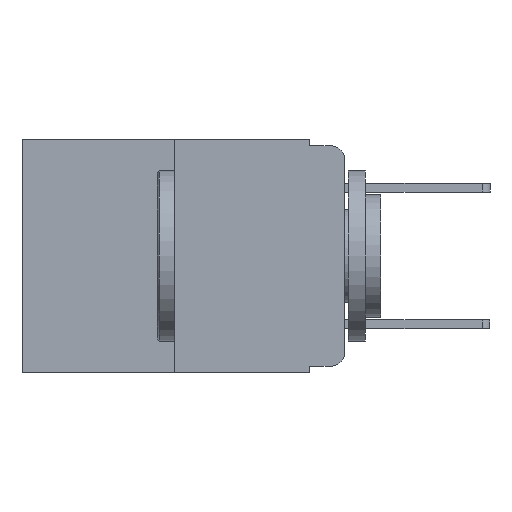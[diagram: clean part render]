
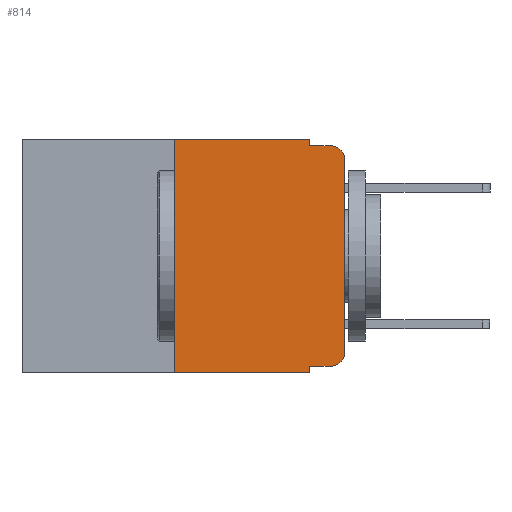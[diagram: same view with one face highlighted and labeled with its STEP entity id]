
A CAD part, left-side view. The second image highlights one B-rep face of the part: STEP entity #814.
In plain terms, the highlighted planar face has unit normal (-1, 0, 0).
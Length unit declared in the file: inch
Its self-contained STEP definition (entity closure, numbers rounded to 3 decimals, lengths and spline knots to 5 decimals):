
#743 = LINE ( 'NONE', #25751, #10506 ) ;
#814 = ADVANCED_FACE ( 'NONE', ( #19289 ), #8830, .F. ) ;
#1158 = CARTESIAN_POINT ( 'NONE',  ( 0., 0.051, 0. ) ) ;
#1259 = EDGE_LOOP ( 'NONE', ( #15015, #2465, #11237, #19828, #19221, #9065, #8106, #18004, #20524, #11002 ) ) ;
#1454 = LINE ( 'NONE', #3544, #11855 ) ;
#2142 = CARTESIAN_POINT ( 'NONE',  ( 0., 0.02, -0.01 ) ) ;
#2465 = ORIENTED_EDGE ( 'NONE', *, *, #15801, .T. ) ;
#2519 = AXIS2_PLACEMENT_3D ( 'NONE', #14335, #8829, #5955 ) ;
#2995 = VERTEX_POINT ( 'NONE', #9192 ) ;
#3394 = CARTESIAN_POINT ( 'NONE',  ( 0., 0., -0.03 ) ) ;
#3544 = CARTESIAN_POINT ( 'NONE',  ( 0., 0.473, -0.343 ) ) ;
#3698 = VERTEX_POINT ( 'NONE', #24868 ) ;
#3718 = EDGE_CURVE ( 'NONE', #3698, #2995, #5769, .T. ) ;
#3882 = VERTEX_POINT ( 'NONE', #15456 ) ;
#4671 = CARTESIAN_POINT ( 'NONE',  ( 0., 0., 0. ) ) ;
#5769 = LINE ( 'NONE', #6802, #15995 ) ;
#5955 = DIRECTION ( 'NONE',  ( 0., 0., -1. ) ) ;
#6186 = CARTESIAN_POINT ( 'NONE',  ( 0., 0.051, -0.01 ) ) ;
#6559 = CARTESIAN_POINT ( 'NONE',  ( 0., 0.473, 0. ) ) ;
#6802 = CARTESIAN_POINT ( 'NONE',  ( 0., 0.25, 0. ) ) ;
#6862 = VECTOR ( 'NONE', #20431, 39.37008 ) ;
#6938 = LINE ( 'NONE', #8905, #11758 ) ;
#7070 = VERTEX_POINT ( 'NONE', #21222 ) ;
#8106 = ORIENTED_EDGE ( 'NONE', *, *, #17532, .T. ) ;
#8263 = CIRCLE ( 'NONE', #25473, 0.02 ) ;
#8444 = EDGE_CURVE ( 'NONE', #3882, #10391, #25463, .T. ) ;
#8630 = DIRECTION ( 'NONE',  ( 0., -1., 0. ) ) ;
#8714 = CARTESIAN_POINT ( 'NONE',  ( 0., 0.02, -0.03 ) ) ;
#8829 = DIRECTION ( 'NONE',  ( 1., 0., 0. ) ) ;
#8830 = PLANE ( 'NONE',  #2519 ) ;
#8876 = DIRECTION ( 'NONE',  ( 0., 0., 1. ) ) ;
#8905 = CARTESIAN_POINT ( 'NONE',  ( 0., 0.051, 0. ) ) ;
#8975 = VERTEX_POINT ( 'NONE', #2142 ) ;
#9019 = CARTESIAN_POINT ( 'NONE',  ( 0., 0.02, -0.313 ) ) ;
#9065 = ORIENTED_EDGE ( 'NONE', *, *, #3718, .F. ) ;
#9192 = CARTESIAN_POINT ( 'NONE',  ( 0., 0.25, 0. ) ) ;
#9265 = VECTOR ( 'NONE', #8630, 39.37008 ) ;
#10391 = VERTEX_POINT ( 'NONE', #3394 ) ;
#10506 = VECTOR ( 'NONE', #19805, 39.37008 ) ;
#10748 = DIRECTION ( 'NONE',  ( 0., 0., -1. ) ) ;
#11002 = ORIENTED_EDGE ( 'NONE', *, *, #15226, .T. ) ;
#11055 = DIRECTION ( 'NONE',  ( 0., 0., -1. ) ) ;
#11237 = ORIENTED_EDGE ( 'NONE', *, *, #21519, .F. ) ;
#11758 = VECTOR ( 'NONE', #15027, 39.37008 ) ;
#11855 = VECTOR ( 'NONE', #19901, 39.37008 ) ;
#12405 = CIRCLE ( 'NONE', #19093, 0.02 ) ;
#14041 = LINE ( 'NONE', #6559, #9265 ) ;
#14154 = VERTEX_POINT ( 'NONE', #25714 ) ;
#14335 = CARTESIAN_POINT ( 'NONE',  ( 0., 0.473, 0. ) ) ;
#15015 = ORIENTED_EDGE ( 'NONE', *, *, #8444, .T. ) ;
#15027 = DIRECTION ( 'NONE',  ( 0., 0., -1. ) ) ;
#15226 = EDGE_CURVE ( 'NONE', #7070, #3882, #8263, .T. ) ;
#15456 = CARTESIAN_POINT ( 'NONE',  ( 0., 0., -0.313 ) ) ;
#15614 = DIRECTION ( 'NONE',  ( 0., 0., -1. ) ) ;
#15642 = LINE ( 'NONE', #1158, #21016 ) ;
#15801 = EDGE_CURVE ( 'NONE', #10391, #8975, #12405, .T. ) ;
#15995 = VECTOR ( 'NONE', #8876, 39.37008 ) ;
#16022 = VERTEX_POINT ( 'NONE', #23510 ) ;
#16437 = LINE ( 'NONE', #6186, #6862 ) ;
#17107 = CARTESIAN_POINT ( 'NONE',  ( 0., 0.051, 0. ) ) ;
#17507 = VERTEX_POINT ( 'NONE', #23784 ) ;
#17532 = EDGE_CURVE ( 'NONE', #3698, #16022, #1454, .T. ) ;
#18004 = ORIENTED_EDGE ( 'NONE', *, *, #26021, .F. ) ;
#18981 = EDGE_CURVE ( 'NONE', #2995, #22466, #14041, .T. ) ;
#19093 = AXIS2_PLACEMENT_3D ( 'NONE', #8714, #22904, #10748 ) ;
#19221 = ORIENTED_EDGE ( 'NONE', *, *, #18981, .F. ) ;
#19289 = FACE_OUTER_BOUND ( 'NONE', #1259, .T. ) ;
#19298 = EDGE_CURVE ( 'NONE', #17507, #7070, #743, .T. ) ;
#19805 = DIRECTION ( 'NONE',  ( 0., -1., 0. ) ) ;
#19828 = ORIENTED_EDGE ( 'NONE', *, *, #20162, .F. ) ;
#19901 = DIRECTION ( 'NONE',  ( 0., -1., 0. ) ) ;
#20162 = EDGE_CURVE ( 'NONE', #22466, #14154, #6938, .T. ) ;
#20431 = DIRECTION ( 'NONE',  ( 0., -1., 0. ) ) ;
#20524 = ORIENTED_EDGE ( 'NONE', *, *, #19298, .T. ) ;
#20984 = DIRECTION ( 'NONE',  ( 0., 0., 1. ) ) ;
#21016 = VECTOR ( 'NONE', #15614, 39.37008 ) ;
#21222 = CARTESIAN_POINT ( 'NONE',  ( 0., 0.02, -0.333 ) ) ;
#21519 = EDGE_CURVE ( 'NONE', #14154, #8975, #16437, .T. ) ;
#22466 = VERTEX_POINT ( 'NONE', #17107 ) ;
#22904 = DIRECTION ( 'NONE',  ( -1., 0., 0. ) ) ;
#23194 = DIRECTION ( 'NONE',  ( -1., 0., 0. ) ) ;
#23510 = CARTESIAN_POINT ( 'NONE',  ( 0., 0.051, -0.343 ) ) ;
#23784 = CARTESIAN_POINT ( 'NONE',  ( 0., 0.051, -0.333 ) ) ;
#24245 = VECTOR ( 'NONE', #20984, 39.37008 ) ;
#24868 = CARTESIAN_POINT ( 'NONE',  ( 0., 0.25, -0.343 ) ) ;
#25463 = LINE ( 'NONE', #4671, #24245 ) ;
#25473 = AXIS2_PLACEMENT_3D ( 'NONE', #9019, #23194, #11055 ) ;
#25714 = CARTESIAN_POINT ( 'NONE',  ( 0., 0.051, -0.01 ) ) ;
#25751 = CARTESIAN_POINT ( 'NONE',  ( 0., 0.051, -0.333 ) ) ;
#26021 = EDGE_CURVE ( 'NONE', #17507, #16022, #15642, .T. ) ;
